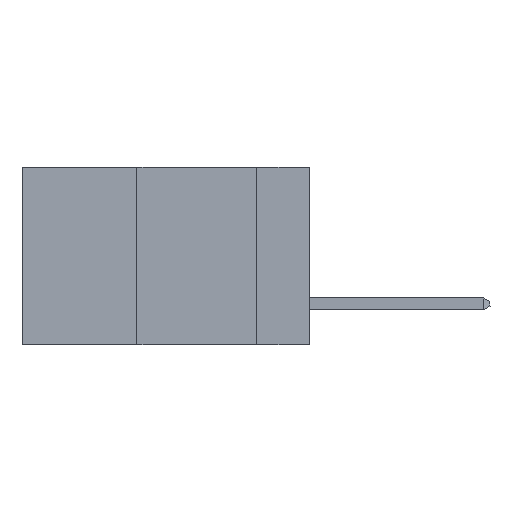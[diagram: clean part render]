
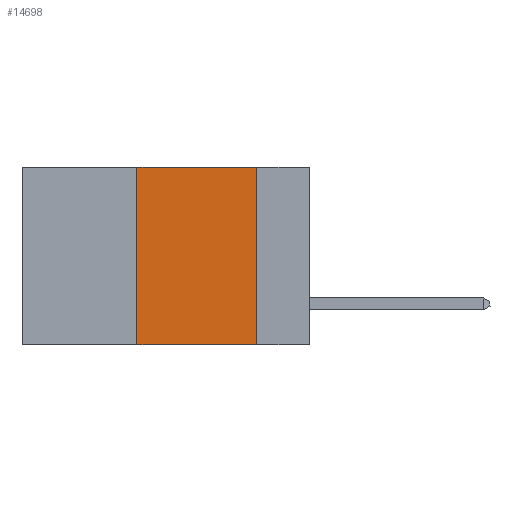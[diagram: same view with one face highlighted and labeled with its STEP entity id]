
A CAD part, left-side view. The second image highlights one B-rep face of the part: STEP entity #14698.
In plain terms, the highlighted planar face has unit normal (-1, 0, 0).
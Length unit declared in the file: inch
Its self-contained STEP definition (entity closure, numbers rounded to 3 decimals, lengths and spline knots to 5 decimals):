
#1261 = ORIENTED_EDGE ( 'NONE', *, *, #9867, .T. ) ;
#3734 = EDGE_CURVE ( 'NONE', #26012, #5210, #12340, .T. ) ;
#4308 = LINE ( 'NONE', #19971, #22061 ) ;
#5210 = VERTEX_POINT ( 'NONE', #9865 ) ;
#7217 = LINE ( 'NONE', #7260, #12943 ) ;
#7260 = CARTESIAN_POINT ( 'NONE',  ( 0., 0.6, 0. ) ) ;
#7291 = LINE ( 'NONE', #22300, #18618 ) ;
#7984 = DIRECTION ( 'NONE',  ( 0., -1., 0. ) ) ;
#8724 = CARTESIAN_POINT ( 'NONE',  ( 0., 0.11, 0. ) ) ;
#8756 = CARTESIAN_POINT ( 'NONE',  ( 0., 0.36, -0.37 ) ) ;
#9199 = EDGE_LOOP ( 'NONE', ( #10428, #14584, #13100, #1261 ) ) ;
#9741 = DIRECTION ( 'NONE',  ( 0., -1., 0. ) ) ;
#9865 = CARTESIAN_POINT ( 'NONE',  ( 0., 0.11, -0.37 ) ) ;
#9867 = EDGE_CURVE ( 'NONE', #19965, #5210, #4308, .T. ) ;
#10056 = DIRECTION ( 'NONE',  ( 0., 0., -1. ) ) ;
#10428 = ORIENTED_EDGE ( 'NONE', *, *, #3734, .F. ) ;
#12340 = LINE ( 'NONE', #29574, #30586 ) ;
#12943 = VECTOR ( 'NONE', #9741, 39.37008 ) ;
#13100 = ORIENTED_EDGE ( 'NONE', *, *, #22136, .F. ) ;
#13156 = CARTESIAN_POINT ( 'NONE',  ( 0., 0.6, 0. ) ) ;
#13485 = VERTEX_POINT ( 'NONE', #19988 ) ;
#14584 = ORIENTED_EDGE ( 'NONE', *, *, #16716, .F. ) ;
#14698 = ADVANCED_FACE ( 'NONE', ( #22820 ), #20241, .F. ) ;
#15523 = DIRECTION ( 'NONE',  ( 0., 0., -1. ) ) ;
#16716 = EDGE_CURVE ( 'NONE', #13485, #26012, #7217, .T. ) ;
#18618 = VECTOR ( 'NONE', #24698, 39.37008 ) ;
#19965 = VERTEX_POINT ( 'NONE', #8756 ) ;
#19971 = CARTESIAN_POINT ( 'NONE',  ( 0., 0.6, -0.37 ) ) ;
#19988 = CARTESIAN_POINT ( 'NONE',  ( 0., 0.36, 0. ) ) ;
#20241 = PLANE ( 'NONE',  #26186 ) ;
#22061 = VECTOR ( 'NONE', #7984, 39.37008 ) ;
#22136 = EDGE_CURVE ( 'NONE', #19965, #13485, #7291, .T. ) ;
#22300 = CARTESIAN_POINT ( 'NONE',  ( 0., 0.36, 0. ) ) ;
#22820 = FACE_OUTER_BOUND ( 'NONE', #9199, .T. ) ;
#24698 = DIRECTION ( 'NONE',  ( 0., 0., 1. ) ) ;
#26012 = VERTEX_POINT ( 'NONE', #8724 ) ;
#26186 = AXIS2_PLACEMENT_3D ( 'NONE', #13156, #29817, #15523 ) ;
#29574 = CARTESIAN_POINT ( 'NONE',  ( 0., 0.11, 0. ) ) ;
#29817 = DIRECTION ( 'NONE',  ( 1., 0., 0. ) ) ;
#30586 = VECTOR ( 'NONE', #10056, 39.37008 ) ;
